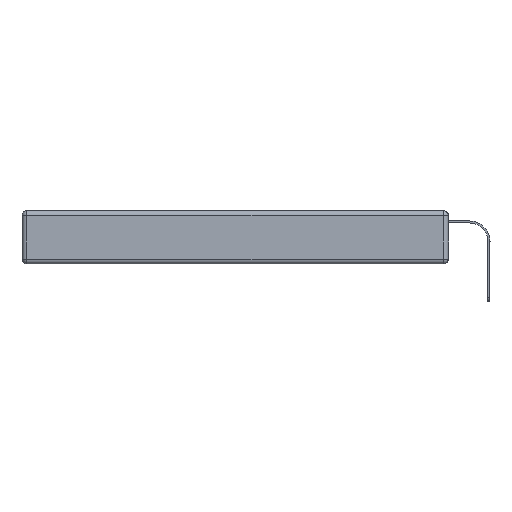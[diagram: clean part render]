
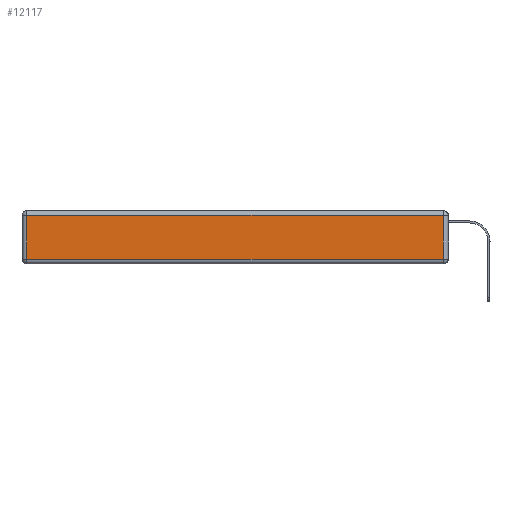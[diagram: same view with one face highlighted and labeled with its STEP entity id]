
A CAD part, left-side view. The second image highlights one B-rep face of the part: STEP entity #12117.
In plain terms, the highlighted planar face has unit normal (-1, 0, 0).
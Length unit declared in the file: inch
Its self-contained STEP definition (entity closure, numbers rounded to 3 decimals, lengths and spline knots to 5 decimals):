
#35 = EDGE_CURVE ( 'NONE', #675, #4606, #2323, .T. ) ;
#198 = DIRECTION ( 'NONE',  ( 0., -1., 0. ) ) ;
#267 = ORIENTED_EDGE ( 'NONE', *, *, #4069, .T. ) ;
#675 = VERTEX_POINT ( 'NONE', #11431 ) ;
#901 = VECTOR ( 'NONE', #11345, 39.37008 ) ;
#1061 = ORIENTED_EDGE ( 'NONE', *, *, #35, .T. ) ;
#1381 = CARTESIAN_POINT ( 'NONE',  ( 0., 2.72, -0.313 ) ) ;
#2323 = LINE ( 'NONE', #6821, #901 ) ;
#2325 = CARTESIAN_POINT ( 'NONE',  ( 0., 0.03, -0.343 ) ) ;
#3098 = AXIS2_PLACEMENT_3D ( 'NONE', #4292, #14603, #11038 ) ;
#3278 = LINE ( 'NONE', #2325, #6959 ) ;
#3904 = EDGE_LOOP ( 'NONE', ( #267, #4883, #6286, #1061 ) ) ;
#4069 = EDGE_CURVE ( 'NONE', #4606, #12998, #12579, .T. ) ;
#4292 = CARTESIAN_POINT ( 'NONE',  ( 0., 0., -0.343 ) ) ;
#4606 = VERTEX_POINT ( 'NONE', #1381 ) ;
#4689 = DIRECTION ( 'NONE',  ( 0., 1., 0. ) ) ;
#4883 = ORIENTED_EDGE ( 'NONE', *, *, #9896, .T. ) ;
#5427 = DIRECTION ( 'NONE',  ( 0., 0., 1. ) ) ;
#6286 = ORIENTED_EDGE ( 'NONE', *, *, #8789, .T. ) ;
#6821 = CARTESIAN_POINT ( 'NONE',  ( 0., 2.72, -0.343 ) ) ;
#6959 = VECTOR ( 'NONE', #5427, 39.37008 ) ;
#7632 = VECTOR ( 'NONE', #4689, 39.37008 ) ;
#8107 = CARTESIAN_POINT ( 'NONE',  ( 0., 0., -0.313 ) ) ;
#8789 = EDGE_CURVE ( 'NONE', #9922, #675, #13739, .T. ) ;
#9016 = VECTOR ( 'NONE', #198, 39.37008 ) ;
#9896 = EDGE_CURVE ( 'NONE', #12998, #9922, #3278, .T. ) ;
#9922 = VERTEX_POINT ( 'NONE', #10016 ) ;
#10016 = CARTESIAN_POINT ( 'NONE',  ( 0., 0.03, -0.03 ) ) ;
#10329 = CARTESIAN_POINT ( 'NONE',  ( 0., 2.75, -0.03 ) ) ;
#11038 = DIRECTION ( 'NONE',  ( 0., 0., 1. ) ) ;
#11175 = PLANE ( 'NONE',  #3098 ) ;
#11345 = DIRECTION ( 'NONE',  ( 0., 0., -1. ) ) ;
#11431 = CARTESIAN_POINT ( 'NONE',  ( 0., 2.72, -0.03 ) ) ;
#12038 = CARTESIAN_POINT ( 'NONE',  ( 0., 0.03, -0.313 ) ) ;
#12117 = ADVANCED_FACE ( 'NONE', ( #12439 ), #11175, .T. ) ;
#12439 = FACE_OUTER_BOUND ( 'NONE', #3904, .T. ) ;
#12579 = LINE ( 'NONE', #8107, #9016 ) ;
#12998 = VERTEX_POINT ( 'NONE', #12038 ) ;
#13739 = LINE ( 'NONE', #10329, #7632 ) ;
#14603 = DIRECTION ( 'NONE',  ( -1., 0., 0. ) ) ;
